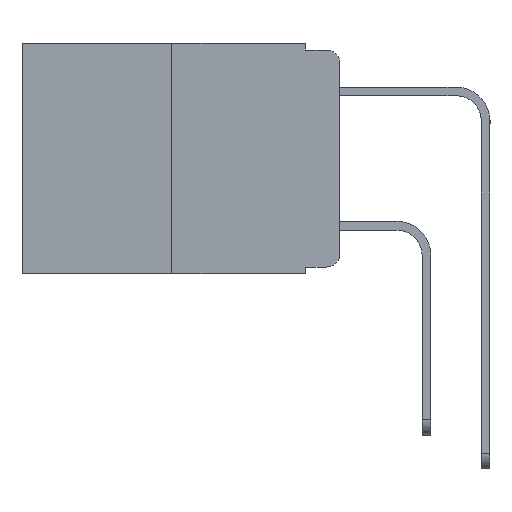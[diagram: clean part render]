
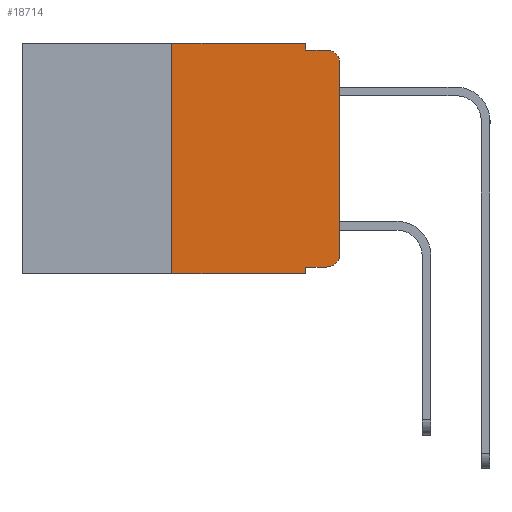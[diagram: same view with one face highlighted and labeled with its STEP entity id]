
A CAD part, left-side view. The second image highlights one B-rep face of the part: STEP entity #18714.
In plain terms, the highlighted planar face has unit normal (-1, 0, 0).
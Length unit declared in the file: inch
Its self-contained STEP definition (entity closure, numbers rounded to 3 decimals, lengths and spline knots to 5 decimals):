
#6 = CARTESIAN_POINT ( 'NONE',  ( 0., 0.051, 0. ) ) ;
#306 = VECTOR ( 'NONE', #15665, 39.37008 ) ;
#365 = CARTESIAN_POINT ( 'NONE',  ( 0., 0.051, -0.01 ) ) ;
#446 = CARTESIAN_POINT ( 'NONE',  ( 0., 0.473, 0. ) ) ;
#489 = VERTEX_POINT ( 'NONE', #7390 ) ;
#538 = EDGE_CURVE ( 'NONE', #11007, #2800, #5514, .T. ) ;
#846 = VERTEX_POINT ( 'NONE', #16029 ) ;
#1119 = CARTESIAN_POINT ( 'NONE',  ( 0., 0.051, 0. ) ) ;
#1121 = VECTOR ( 'NONE', #3510, 39.37008 ) ;
#1178 = CARTESIAN_POINT ( 'NONE',  ( 0., 0.25, -0.343 ) ) ;
#1335 = CARTESIAN_POINT ( 'NONE',  ( 0., 0., 0. ) ) ;
#1491 = VECTOR ( 'NONE', #7637, 39.37008 ) ;
#1523 = CIRCLE ( 'NONE', #18927, 0.02 ) ;
#1820 = EDGE_CURVE ( 'NONE', #12345, #11007, #7459, .T. ) ;
#2148 = EDGE_CURVE ( 'NONE', #6949, #7148, #4748, .T. ) ;
#2800 = VERTEX_POINT ( 'NONE', #17776 ) ;
#3235 = CARTESIAN_POINT ( 'NONE',  ( 0., 0.051, -0.343 ) ) ;
#3255 = DIRECTION ( 'NONE',  ( 0., -1., 0. ) ) ;
#3365 = CARTESIAN_POINT ( 'NONE',  ( 0., 0.473, 0. ) ) ;
#3510 = DIRECTION ( 'NONE',  ( 0., 0., -1. ) ) ;
#4126 = EDGE_LOOP ( 'NONE', ( #9785, #17525, #10253, #17979, #6588, #14601, #18420, #7064, #18877, #11671 ) ) ;
#4748 = LINE ( 'NONE', #8302, #12473 ) ;
#4849 = DIRECTION ( 'NONE',  ( -1., 0., 0. ) ) ;
#5514 = LINE ( 'NONE', #10009, #1121 ) ;
#5605 = LINE ( 'NONE', #11090, #14608 ) ;
#6127 = EDGE_CURVE ( 'NONE', #6798, #846, #10223, .T. ) ;
#6588 = ORIENTED_EDGE ( 'NONE', *, *, #1820, .F. ) ;
#6798 = VERTEX_POINT ( 'NONE', #8664 ) ;
#6809 = PLANE ( 'NONE',  #15120 ) ;
#6949 = VERTEX_POINT ( 'NONE', #1178 ) ;
#7064 = ORIENTED_EDGE ( 'NONE', *, *, #13048, .F. ) ;
#7073 = EDGE_CURVE ( 'NONE', #17942, #489, #12668, .T. ) ;
#7148 = VERTEX_POINT ( 'NONE', #3235 ) ;
#7390 = CARTESIAN_POINT ( 'NONE',  ( 0., 0.02, -0.333 ) ) ;
#7459 = LINE ( 'NONE', #3365, #14082 ) ;
#7623 = EDGE_CURVE ( 'NONE', #489, #16298, #1523, .T. ) ;
#7637 = DIRECTION ( 'NONE',  ( 0., 0., 1. ) ) ;
#7956 = DIRECTION ( 'NONE',  ( -1., 0., 0. ) ) ;
#8082 = CARTESIAN_POINT ( 'NONE',  ( 0., 0.051, -0.333 ) ) ;
#8302 = CARTESIAN_POINT ( 'NONE',  ( 0., 0.473, -0.343 ) ) ;
#8391 = DIRECTION ( 'NONE',  ( 0., 0., -1. ) ) ;
#8664 = CARTESIAN_POINT ( 'NONE',  ( 0., 0., -0.03 ) ) ;
#8732 = LINE ( 'NONE', #365, #306 ) ;
#9357 = DIRECTION ( 'NONE',  ( 0., -1., 0. ) ) ;
#9785 = ORIENTED_EDGE ( 'NONE', *, *, #14110, .T. ) ;
#10009 = CARTESIAN_POINT ( 'NONE',  ( 0., 0.051, 0. ) ) ;
#10223 = CIRCLE ( 'NONE', #12041, 0.02 ) ;
#10253 = ORIENTED_EDGE ( 'NONE', *, *, #18677, .F. ) ;
#11007 = VERTEX_POINT ( 'NONE', #6 ) ;
#11064 = LINE ( 'NONE', #1119, #14478 ) ;
#11090 = CARTESIAN_POINT ( 'NONE',  ( 0., 0.25, 0. ) ) ;
#11579 = CARTESIAN_POINT ( 'NONE',  ( 0., 0.25, 0. ) ) ;
#11590 = EDGE_CURVE ( 'NONE', #6949, #12345, #5605, .T. ) ;
#11671 = ORIENTED_EDGE ( 'NONE', *, *, #7623, .T. ) ;
#12041 = AXIS2_PLACEMENT_3D ( 'NONE', #14007, #4849, #15437 ) ;
#12345 = VERTEX_POINT ( 'NONE', #11579 ) ;
#12473 = VECTOR ( 'NONE', #15603, 39.37008 ) ;
#12668 = LINE ( 'NONE', #19539, #13591 ) ;
#13048 = EDGE_CURVE ( 'NONE', #17942, #7148, #11064, .T. ) ;
#13292 = LINE ( 'NONE', #1335, #1491 ) ;
#13591 = VECTOR ( 'NONE', #9357, 39.37008 ) ;
#14007 = CARTESIAN_POINT ( 'NONE',  ( 0., 0.02, -0.03 ) ) ;
#14082 = VECTOR ( 'NONE', #3255, 39.37008 ) ;
#14110 = EDGE_CURVE ( 'NONE', #16298, #6798, #13292, .T. ) ;
#14478 = VECTOR ( 'NONE', #19300, 39.37008 ) ;
#14601 = ORIENTED_EDGE ( 'NONE', *, *, #11590, .F. ) ;
#14608 = VECTOR ( 'NONE', #16906, 39.37008 ) ;
#15120 = AXIS2_PLACEMENT_3D ( 'NONE', #446, #17224, #8391 ) ;
#15437 = DIRECTION ( 'NONE',  ( 0., 0., -1. ) ) ;
#15603 = DIRECTION ( 'NONE',  ( 0., -1., 0. ) ) ;
#15665 = DIRECTION ( 'NONE',  ( 0., -1., 0. ) ) ;
#15676 = FACE_OUTER_BOUND ( 'NONE', #4126, .T. ) ;
#16029 = CARTESIAN_POINT ( 'NONE',  ( 0., 0.02, -0.01 ) ) ;
#16298 = VERTEX_POINT ( 'NONE', #17275 ) ;
#16830 = CARTESIAN_POINT ( 'NONE',  ( 0., 0.02, -0.313 ) ) ;
#16906 = DIRECTION ( 'NONE',  ( 0., 0., 1. ) ) ;
#17224 = DIRECTION ( 'NONE',  ( 1., 0., 0. ) ) ;
#17275 = CARTESIAN_POINT ( 'NONE',  ( 0., 0., -0.313 ) ) ;
#17525 = ORIENTED_EDGE ( 'NONE', *, *, #6127, .T. ) ;
#17776 = CARTESIAN_POINT ( 'NONE',  ( 0., 0.051, -0.01 ) ) ;
#17942 = VERTEX_POINT ( 'NONE', #8082 ) ;
#17979 = ORIENTED_EDGE ( 'NONE', *, *, #538, .F. ) ;
#18269 = DIRECTION ( 'NONE',  ( 0., 0., -1. ) ) ;
#18420 = ORIENTED_EDGE ( 'NONE', *, *, #2148, .T. ) ;
#18677 = EDGE_CURVE ( 'NONE', #2800, #846, #8732, .T. ) ;
#18714 = ADVANCED_FACE ( 'NONE', ( #15676 ), #6809, .F. ) ;
#18877 = ORIENTED_EDGE ( 'NONE', *, *, #7073, .T. ) ;
#18927 = AXIS2_PLACEMENT_3D ( 'NONE', #16830, #7956, #18269 ) ;
#19300 = DIRECTION ( 'NONE',  ( 0., 0., -1. ) ) ;
#19539 = CARTESIAN_POINT ( 'NONE',  ( 0., 0.051, -0.333 ) ) ;
